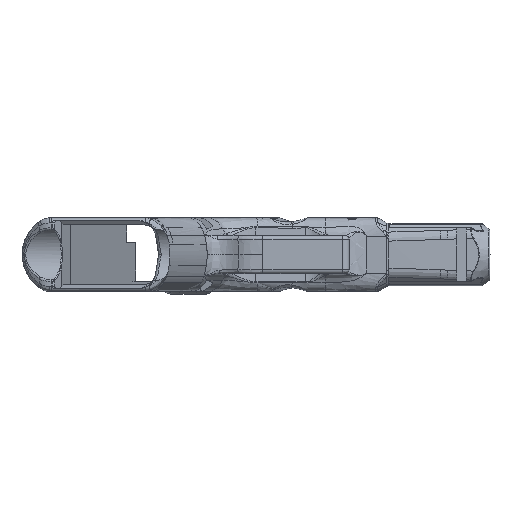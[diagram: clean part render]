
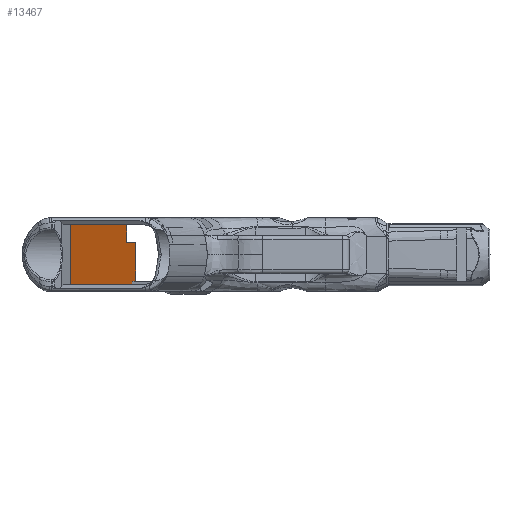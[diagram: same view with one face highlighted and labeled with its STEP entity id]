
A CAD part, front view. The second image highlights one B-rep face of the part: STEP entity #13467.
In plain terms, the highlighted planar face has unit normal (0.951, -0.309, 0).
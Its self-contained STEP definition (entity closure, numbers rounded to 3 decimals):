
#1414=FACE_OUTER_BOUND('',#2132,.T.);
#2132=EDGE_LOOP('',(#11922,#11923,#11924,#11925,#11926,#11927,#11928,#11929));
#3531=LINE('',#25835,#4267);
#3636=LINE('',#28292,#4372);
#3654=LINE('',#29448,#4390);
#3707=LINE('',#37780,#4443);
#3721=LINE('',#37968,#4457);
#3743=LINE('',#40042,#4479);
#3744=LINE('',#40108,#4480);
#3753=LINE('',#40608,#4489);
#4267=VECTOR('',#15528,10.);
#4372=VECTOR('',#15811,10.);
#4390=VECTOR('',#15909,10.);
#4443=VECTOR('',#16192,10.);
#4457=VECTOR('',#16212,10.);
#4479=VECTOR('',#16296,10.);
#4480=VECTOR('',#16303,10.);
#4489=VECTOR('',#16354,10.);
#5177=VERTEX_POINT('',#25833);
#5178=VERTEX_POINT('',#25834);
#5357=VERTEX_POINT('',#28289);
#5358=VERTEX_POINT('',#28291);
#5564=VERTEX_POINT('',#37779);
#5573=VERTEX_POINT('',#37933);
#5577=VERTEX_POINT('',#37966);
#5624=VERTEX_POINT('',#40107);
#6654=EDGE_CURVE('',#5177,#5178,#3531,.T.);
#6888=EDGE_CURVE('',#5358,#5357,#3636,.T.);
#6966=EDGE_CURVE('',#5177,#5357,#3654,.T.);
#7223=EDGE_CURVE('',#5358,#5564,#3707,.T.);
#7243=EDGE_CURVE('',#5577,#5573,#3721,.T.);
#7310=EDGE_CURVE('',#5564,#5577,#3743,.T.);
#7313=EDGE_CURVE('',#5573,#5624,#3744,.T.);
#7342=EDGE_CURVE('',#5624,#5178,#3753,.T.);
#11922=ORIENTED_EDGE('',*,*,#6966,.F.);
#11923=ORIENTED_EDGE('',*,*,#6654,.T.);
#11924=ORIENTED_EDGE('',*,*,#7342,.F.);
#11925=ORIENTED_EDGE('',*,*,#7313,.F.);
#11926=ORIENTED_EDGE('',*,*,#7243,.F.);
#11927=ORIENTED_EDGE('',*,*,#7310,.F.);
#11928=ORIENTED_EDGE('',*,*,#7223,.F.);
#11929=ORIENTED_EDGE('',*,*,#6888,.T.);
#12169=PLANE('',#14499);
#13467=ADVANCED_FACE('',(#1414),#12169,.F.);
#14499=AXIS2_PLACEMENT_3D('',#54978,#17235,#17236);
#15528=DIRECTION('',(0.309,0.951,0.));
#15811=DIRECTION('',(-0.309,-0.951,0.));
#15909=DIRECTION('',(0.,0.,1.));
#16192=DIRECTION('',(0.,0.,-1.));
#16212=DIRECTION('',(0.,0.,-1.));
#16296=DIRECTION('',(0.309,0.951,0.));
#16303=DIRECTION('',(-0.309,-0.951,0.));
#16354=DIRECTION('',(0.,0.,-1.));
#17235=DIRECTION('center_axis',(-0.951,0.309,0.));
#17236=DIRECTION('ref_axis',(0.,0.,
1.));
#25833=CARTESIAN_POINT('',(8.112,-79.915,-11.75));
#25834=CARTESIAN_POINT('',(32.169,-5.875,-11.75));
#25835=CARTESIAN_POINT('',(2.312,-97.765,-11.75));
#28289=CARTESIAN_POINT('',(8.112,-79.915,11.75));
#28291=CARTESIAN_POINT('',(30.049,-12.4,11.75));
#28292=CARTESIAN_POINT('',(2.312,-97.765,11.75));
#29448=CARTESIAN_POINT('',(8.112,-79.915,-13.075));
#37779=CARTESIAN_POINT('',(30.049,-12.4,4.75));
#37780=CARTESIAN_POINT('',(30.049,-12.4,2.982));
#37933=CARTESIAN_POINT('',(33.591,-1.5,-10.375));
#37966=CARTESIAN_POINT('',(33.591,-1.5,4.75));
#37968=CARTESIAN_POINT('',(33.591,-1.5,-5.875));
#40042=CARTESIAN_POINT('',(18.86,-46.836,4.75));
#40107=CARTESIAN_POINT('',(32.169,-5.875,-10.375));
#40108=CARTESIAN_POINT('',(17.241,-51.82,-10.375));
#40608=CARTESIAN_POINT('',(32.169,-5.875,-5.875));
#54978=CARTESIAN_POINT('Origin',(2.312,-97.765,-11.75));
